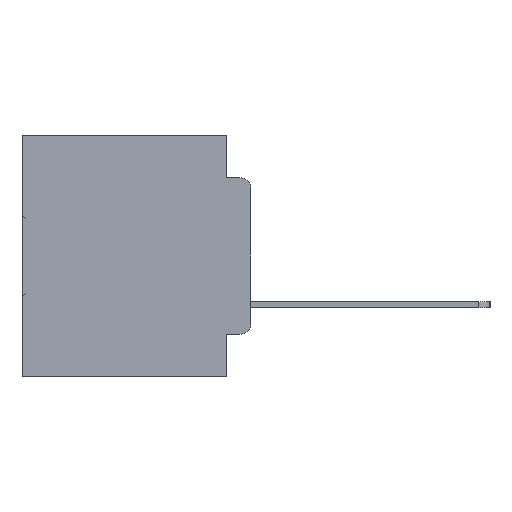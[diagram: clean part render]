
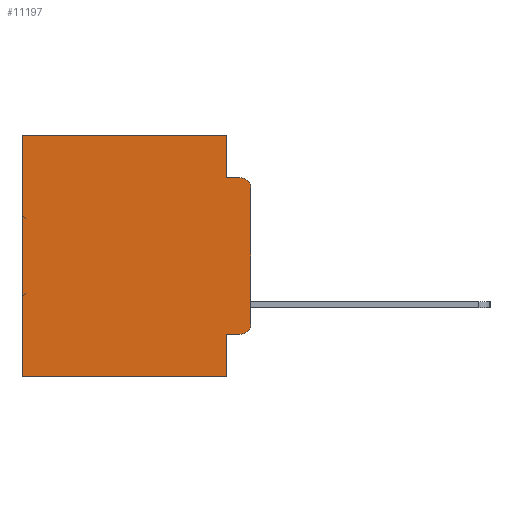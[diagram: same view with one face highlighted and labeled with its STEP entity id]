
A CAD part, left-side view. The second image highlights one B-rep face of the part: STEP entity #11197.
In plain terms, the highlighted planar face has unit normal (-1, 0, 0).
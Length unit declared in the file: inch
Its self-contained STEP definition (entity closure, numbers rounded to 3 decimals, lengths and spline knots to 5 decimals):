
#219 = LINE ( 'NONE', #12705, #34990 ) ;
#750 = CARTESIAN_POINT ( 'NONE',  ( 0.298, 0.02, -0.0885 ) ) ;
#1240 = CARTESIAN_POINT ( 'NONE',  ( 0.298, 0.473, 0. ) ) ;
#1910 = CARTESIAN_POINT ( 'NONE',  ( 0.298, 0.051, 0. ) ) ;
#2287 = DIRECTION ( 'NONE',  ( -1., 0., 0. ) ) ;
#3717 = VECTOR ( 'NONE', #7201, 39.37008 ) ;
#3760 = VERTEX_POINT ( 'NONE', #1240 ) ;
#4891 = CARTESIAN_POINT ( 'NONE',  ( 0.298, 0.051, -0.4115 ) ) ;
#5183 = EDGE_CURVE ( 'NONE', #19086, #34275, #14996, .T. ) ;
#5578 = VECTOR ( 'NONE', #36012, 39.37008 ) ;
#5601 = ORIENTED_EDGE ( 'NONE', *, *, #11346, .F. ) ;
#5623 = EDGE_CURVE ( 'NONE', #27421, #33387, #20786, .T. ) ;
#5751 = ORIENTED_EDGE ( 'NONE', *, *, #7328, .T. ) ;
#6715 = LINE ( 'NONE', #30073, #3717 ) ;
#6757 = ORIENTED_EDGE ( 'NONE', *, *, #5183, .F. ) ;
#7007 = ORIENTED_EDGE ( 'NONE', *, *, #34511, .F. ) ;
#7201 = DIRECTION ( 'NONE',  ( 0., 1., 0. ) ) ;
#7234 = ORIENTED_EDGE ( 'NONE', *, *, #29351, .T. ) ;
#7328 = EDGE_CURVE ( 'NONE', #25257, #34275, #31866, .T. ) ;
#8706 = ORIENTED_EDGE ( 'NONE', *, *, #32755, .T. ) ;
#8744 = ORIENTED_EDGE ( 'NONE', *, *, #5623, .F. ) ;
#9196 = ORIENTED_EDGE ( 'NONE', *, *, #30981, .F. ) ;
#9281 = ORIENTED_EDGE ( 'NONE', *, *, #27352, .T. ) ;
#9547 = ORIENTED_EDGE ( 'NONE', *, *, #25484, .T. ) ;
#10270 = CARTESIAN_POINT ( 'NONE',  ( 0.298, 0.02, -0.3915 ) ) ;
#11006 = DIRECTION ( 'NONE',  ( 0., -1., 0. ) ) ;
#11197 = ADVANCED_FACE ( 'NONE', ( #13314 ), #28313, .F. ) ;
#11246 = DIRECTION ( 'NONE',  ( 0., 1., 0. ) ) ;
#11346 = EDGE_CURVE ( 'NONE', #25257, #17343, #219, .T. ) ;
#12074 = CARTESIAN_POINT ( 'NONE',  ( 0.298, 0.051, -0.4115 ) ) ;
#12536 = VECTOR ( 'NONE', #30591, 39.37008 ) ;
#12699 = CARTESIAN_POINT ( 'NONE',  ( 0.298, 0.02, -0.4115 ) ) ;
#12705 = CARTESIAN_POINT ( 'NONE',  ( 0.298, 0., 0. ) ) ;
#13222 = DIRECTION ( 'NONE',  ( 0., 0., -1. ) ) ;
#13314 = FACE_OUTER_BOUND ( 'NONE', #28770, .T. ) ;
#14057 = LINE ( 'NONE', #1910, #35232 ) ;
#14270 = DIRECTION ( 'NONE',  ( 0., 0., -1. ) ) ;
#14439 = AXIS2_PLACEMENT_3D ( 'NONE', #20222, #2287, #23055 ) ;
#14835 = VECTOR ( 'NONE', #25348, 39.37008 ) ;
#14996 = LINE ( 'NONE', #28077, #36053 ) ;
#15630 = VERTEX_POINT ( 'NONE', #16885 ) ;
#16526 = VERTEX_POINT ( 'NONE', #12074 ) ;
#16885 = CARTESIAN_POINT ( 'NONE',  ( 0.298, 0.051, 0. ) ) ;
#16977 = DIRECTION ( 'NONE',  ( 0., 0., -1. ) ) ;
#17097 = CARTESIAN_POINT ( 'NONE',  ( 0.298, 0., -0.5 ) ) ;
#17343 = VERTEX_POINT ( 'NONE', #21116 ) ;
#17670 = CARTESIAN_POINT ( 'NONE',  ( 0.298, 0.051, -0.5 ) ) ;
#19086 = VERTEX_POINT ( 'NONE', #27450 ) ;
#19743 = CARTESIAN_POINT ( 'NONE',  ( 0.298, 0.051, 0. ) ) ;
#19883 = VECTOR ( 'NONE', #11246, 39.37008 ) ;
#20222 = CARTESIAN_POINT ( 'NONE',  ( 0.298, 0.02, -0.1085 ) ) ;
#20786 = LINE ( 'NONE', #17097, #19883 ) ;
#21116 = CARTESIAN_POINT ( 'NONE',  ( 0.298, 0., -0.3915 ) ) ;
#22150 = LINE ( 'NONE', #19743, #5578 ) ;
#23055 = DIRECTION ( 'NONE',  ( 0., 0., -1. ) ) ;
#25257 = VERTEX_POINT ( 'NONE', #28000 ) ;
#25348 = DIRECTION ( 'NONE',  ( 0., -1., 0. ) ) ;
#25407 = CARTESIAN_POINT ( 'NONE',  ( 0.298, 0.473, -0.5 ) ) ;
#25424 = CARTESIAN_POINT ( 'NONE',  ( 0.298, 0., 0. ) ) ;
#25484 = EDGE_CURVE ( 'NONE', #28347, #17343, #30445, .T. ) ;
#27352 = EDGE_CURVE ( 'NONE', #16526, #28347, #29759, .T. ) ;
#27421 = VERTEX_POINT ( 'NONE', #17670 ) ;
#27450 = CARTESIAN_POINT ( 'NONE',  ( 0.298, 0.051, -0.0885 ) ) ;
#27761 = AXIS2_PLACEMENT_3D ( 'NONE', #25424, #31044, #14270 ) ;
#27860 = CARTESIAN_POINT ( 'NONE',  ( 0.298, 0.473, 0. ) ) ;
#28000 = CARTESIAN_POINT ( 'NONE',  ( 0.298, 0., -0.1085 ) ) ;
#28077 = CARTESIAN_POINT ( 'NONE',  ( 0.298, 0.051, -0.0885 ) ) ;
#28313 = PLANE ( 'NONE',  #27761 ) ;
#28347 = VERTEX_POINT ( 'NONE', #12699 ) ;
#28770 = EDGE_LOOP ( 'NONE', ( #5601, #5751, #6757, #7007, #7234, #8706, #8744, #9196, #9281, #9547 ) ) ;
#29351 = EDGE_CURVE ( 'NONE', #15630, #3760, #6715, .T. ) ;
#29759 = LINE ( 'NONE', #4891, #14835 ) ;
#30073 = CARTESIAN_POINT ( 'NONE',  ( 0.298, 0., 0. ) ) ;
#30092 = DIRECTION ( 'NONE',  ( -1., 0., 0. ) ) ;
#30445 = CIRCLE ( 'NONE', #35372, 0.02 ) ;
#30591 = DIRECTION ( 'NONE',  ( 0., 0., -1. ) ) ;
#30981 = EDGE_CURVE ( 'NONE', #16526, #27421, #14057, .T. ) ;
#31044 = DIRECTION ( 'NONE',  ( 1., 0., 0. ) ) ;
#31866 = CIRCLE ( 'NONE', #14439, 0.02 ) ;
#32755 = EDGE_CURVE ( 'NONE', #3760, #33387, #34732, .T. ) ;
#33387 = VERTEX_POINT ( 'NONE', #25407 ) ;
#34275 = VERTEX_POINT ( 'NONE', #750 ) ;
#34511 = EDGE_CURVE ( 'NONE', #15630, #19086, #22150, .T. ) ;
#34732 = LINE ( 'NONE', #27860, #12536 ) ;
#34920 = DIRECTION ( 'NONE',  ( 0., 0., -1. ) ) ;
#34990 = VECTOR ( 'NONE', #34920, 39.37008 ) ;
#35232 = VECTOR ( 'NONE', #16977, 39.37008 ) ;
#35372 = AXIS2_PLACEMENT_3D ( 'NONE', #10270, #30092, #13222 ) ;
#36012 = DIRECTION ( 'NONE',  ( 0., 0., -1. ) ) ;
#36053 = VECTOR ( 'NONE', #11006, 39.37008 ) ;
